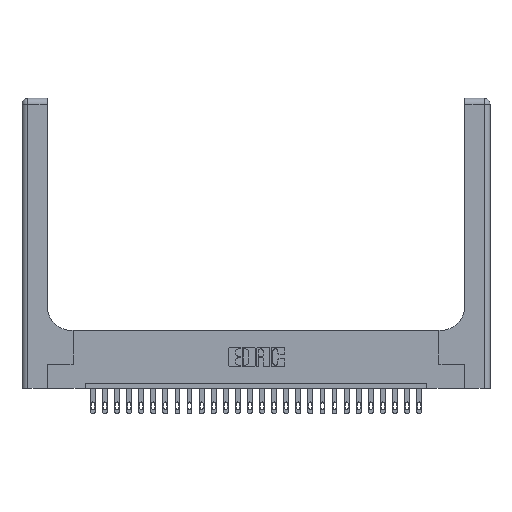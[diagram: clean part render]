
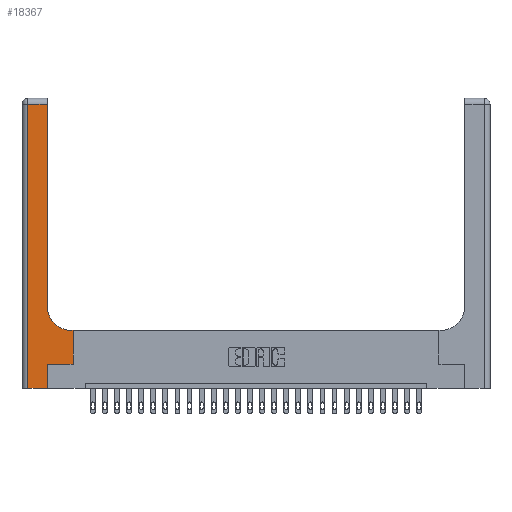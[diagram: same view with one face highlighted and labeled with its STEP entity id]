
A CAD part, top view. The second image highlights one B-rep face of the part: STEP entity #18367.
In plain terms, the highlighted planar face has unit normal (0, 0, 1).
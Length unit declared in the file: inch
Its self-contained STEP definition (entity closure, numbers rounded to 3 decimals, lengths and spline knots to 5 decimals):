
#529 = CARTESIAN_POINT ( 'NONE',  ( 0.528, 0.25, 0.37 ) ) ;
#689 = EDGE_LOOP ( 'NONE', ( #21801, #15948, #1473, #3611, #6723, #22095, #13009, #8727, #5193 ) ) ;
#822 = VECTOR ( 'NONE', #11590, 39.37008 ) ;
#875 = EDGE_CURVE ( 'NONE', #3024, #7305, #13684, .T. ) ;
#896 = LINE ( 'NONE', #18226, #17154 ) ;
#1473 = ORIENTED_EDGE ( 'NONE', *, *, #17136, .T. ) ;
#2165 = CARTESIAN_POINT ( 'NONE',  ( 0.26, 0.85, 0.37 ) ) ;
#2531 = PLANE ( 'NONE',  #18086 ) ;
#2900 = DIRECTION ( 'NONE',  ( 0., -1., 0. ) ) ;
#3022 = EDGE_CURVE ( 'NONE', #15925, #13713, #896, .T. ) ;
#3024 = VERTEX_POINT ( 'NONE', #4422 ) ;
#3362 = VECTOR ( 'NONE', #4002, 39.37008 ) ;
#3611 = ORIENTED_EDGE ( 'NONE', *, *, #18250, .T. ) ;
#4002 = DIRECTION ( 'NONE',  ( 1., 0., 0. ) ) ;
#4028 = LINE ( 'NONE', #15693, #7327 ) ;
#4375 = VERTEX_POINT ( 'NONE', #6464 ) ;
#4422 = CARTESIAN_POINT ( 'NONE',  ( 0.528, 0.6, 0.37 ) ) ;
#4789 = CARTESIAN_POINT ( 'NONE',  ( 0.265, 0., 0.37 ) ) ;
#4808 = VERTEX_POINT ( 'NONE', #2165 ) ;
#5193 = ORIENTED_EDGE ( 'NONE', *, *, #12482, .T. ) ;
#5239 = EDGE_CURVE ( 'NONE', #4808, #4375, #10059, .T. ) ;
#6464 = CARTESIAN_POINT ( 'NONE',  ( 0.26, 2.94, 0.37 ) ) ;
#6723 = ORIENTED_EDGE ( 'NONE', *, *, #3022, .T. ) ;
#6972 = CARTESIAN_POINT ( 'NONE',  ( 0.26, 0.6, 0.37 ) ) ;
#7305 = VERTEX_POINT ( 'NONE', #23047 ) ;
#7327 = VECTOR ( 'NONE', #23469, 39.37008 ) ;
#7448 = CARTESIAN_POINT ( 'NONE',  ( 0., 2.94, 0.37 ) ) ;
#8005 = VECTOR ( 'NONE', #2900, 39.37008 ) ;
#8169 = DIRECTION ( 'NONE',  ( 0., 1., 0. ) ) ;
#8186 = LINE ( 'NONE', #21239, #822 ) ;
#8433 = CARTESIAN_POINT ( 'NONE',  ( 0.06, 2.94, 0.37 ) ) ;
#8484 = EDGE_CURVE ( 'NONE', #13713, #18341, #17549, .T. ) ;
#8727 = ORIENTED_EDGE ( 'NONE', *, *, #875, .T. ) ;
#9467 = VECTOR ( 'NONE', #20641, 39.37008 ) ;
#9574 = EDGE_CURVE ( 'NONE', #4375, #15845, #13002, .T. ) ;
#9934 = AXIS2_PLACEMENT_3D ( 'NONE', #12376, #16506, #20019 ) ;
#10059 = LINE ( 'NONE', #13943, #23754 ) ;
#11590 = DIRECTION ( 'NONE',  ( 1., 0., 0. ) ) ;
#12097 = DIRECTION ( 'NONE',  ( 0., 1., 0. ) ) ;
#12336 = DIRECTION ( 'NONE',  ( 0., 0., -1. ) ) ;
#12376 = CARTESIAN_POINT ( 'NONE',  ( 0.51, 0.85, 0.37 ) ) ;
#12466 = FACE_OUTER_BOUND ( 'NONE', #689, .T. ) ;
#12482 = EDGE_CURVE ( 'NONE', #7305, #4808, #13539, .T. ) ;
#13002 = LINE ( 'NONE', #7448, #9467 ) ;
#13009 = ORIENTED_EDGE ( 'NONE', *, *, #20685, .T. ) ;
#13138 = CARTESIAN_POINT ( 'NONE',  ( 0.06, 0., 0.37 ) ) ;
#13539 = CIRCLE ( 'NONE', #9934, 0.25 ) ;
#13674 = CARTESIAN_POINT ( 'NONE',  ( 0.265, 0.25, 0.37 ) ) ;
#13684 = LINE ( 'NONE', #6972, #15472 ) ;
#13713 = VERTEX_POINT ( 'NONE', #19778 ) ;
#13943 = CARTESIAN_POINT ( 'NONE',  ( 0.26, 3., 0.37 ) ) ;
#14337 = DIRECTION ( 'NONE',  ( -1., 0., 0. ) ) ;
#14458 = CARTESIAN_POINT ( 'NONE',  ( 0.06, 3., 0.37 ) ) ;
#15472 = VECTOR ( 'NONE', #23923, 39.37008 ) ;
#15693 = CARTESIAN_POINT ( 'NONE',  ( 0.528, 0.25, 0.37 ) ) ;
#15845 = VERTEX_POINT ( 'NONE', #8433 ) ;
#15925 = VERTEX_POINT ( 'NONE', #4789 ) ;
#15948 = ORIENTED_EDGE ( 'NONE', *, *, #9574, .T. ) ;
#16506 = DIRECTION ( 'NONE',  ( 0., 0., -1. ) ) ;
#17136 = EDGE_CURVE ( 'NONE', #15845, #23978, #23620, .T. ) ;
#17154 = VECTOR ( 'NONE', #12097, 39.37008 ) ;
#17549 = LINE ( 'NONE', #13674, #3362 ) ;
#18086 = AXIS2_PLACEMENT_3D ( 'NONE', #21748, #12336, #14337 ) ;
#18226 = CARTESIAN_POINT ( 'NONE',  ( 0.265, 0., 0.37 ) ) ;
#18250 = EDGE_CURVE ( 'NONE', #23978, #15925, #8186, .T. ) ;
#18341 = VERTEX_POINT ( 'NONE', #529 ) ;
#18367 = ADVANCED_FACE ( 'NONE', ( #12466 ), #2531, .F. ) ;
#19778 = CARTESIAN_POINT ( 'NONE',  ( 0.265, 0.25, 0.37 ) ) ;
#20019 = DIRECTION ( 'NONE',  ( 1., 0., 0. ) ) ;
#20641 = DIRECTION ( 'NONE',  ( -1., 0., 0. ) ) ;
#20685 = EDGE_CURVE ( 'NONE', #18341, #3024, #4028, .T. ) ;
#21239 = CARTESIAN_POINT ( 'NONE',  ( 0., 0., 0.37 ) ) ;
#21748 = CARTESIAN_POINT ( 'NONE',  ( 0., 3., 0.37 ) ) ;
#21801 = ORIENTED_EDGE ( 'NONE', *, *, #5239, .T. ) ;
#22095 = ORIENTED_EDGE ( 'NONE', *, *, #8484, .T. ) ;
#23047 = CARTESIAN_POINT ( 'NONE',  ( 0.51, 0.6, 0.37 ) ) ;
#23469 = DIRECTION ( 'NONE',  ( 0., 1., 0. ) ) ;
#23620 = LINE ( 'NONE', #14458, #8005 ) ;
#23754 = VECTOR ( 'NONE', #8169, 39.37008 ) ;
#23923 = DIRECTION ( 'NONE',  ( -1., 0., 0. ) ) ;
#23978 = VERTEX_POINT ( 'NONE', #13138 ) ;
